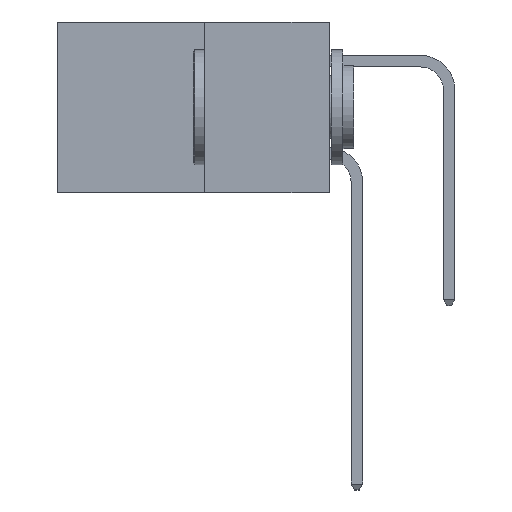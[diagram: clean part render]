
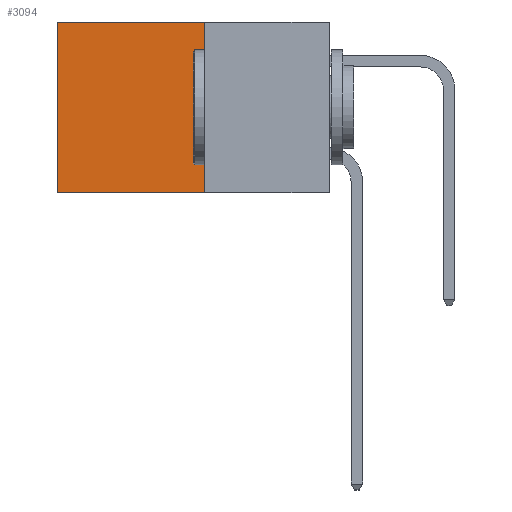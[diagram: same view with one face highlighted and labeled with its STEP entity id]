
A CAD part, left-side view. The second image highlights one B-rep face of the part: STEP entity #3094.
In plain terms, the highlighted planar face has unit normal (-1, 0, 0).
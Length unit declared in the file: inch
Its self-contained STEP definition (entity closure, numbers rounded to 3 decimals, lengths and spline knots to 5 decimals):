
#501 = DIRECTION ( 'NONE',  ( 0., 0., -1. ) ) ;
#2658 = ORIENTED_EDGE ( 'NONE', *, *, #6860, .T. ) ;
#2930 = VECTOR ( 'NONE', #501, 39.37008 ) ;
#3094 = ADVANCED_FACE ( 'NONE', ( #4518 ), #5995, .F. ) ;
#3196 = VERTEX_POINT ( 'NONE', #6927 ) ;
#3282 = LINE ( 'NONE', #6201, #2930 ) ;
#3519 = ORIENTED_EDGE ( 'NONE', *, *, #13353, .F. ) ;
#4063 = CARTESIAN_POINT ( 'NONE',  ( 0.277, 0.27, -0.37 ) ) ;
#4080 = CARTESIAN_POINT ( 'NONE',  ( 0.277, 0.27, 0. ) ) ;
#4437 = EDGE_LOOP ( 'NONE', ( #2658, #3519, #10215, #11850 ) ) ;
#4518 = FACE_OUTER_BOUND ( 'NONE', #4437, .T. ) ;
#4732 = DIRECTION ( 'NONE',  ( 0., 0., -1. ) ) ;
#4769 = DIRECTION ( 'NONE',  ( 1., 0., 0. ) ) ;
#4924 = LINE ( 'NONE', #4063, #14183 ) ;
#5316 = LINE ( 'NONE', #4080, #8425 ) ;
#5400 = VERTEX_POINT ( 'NONE', #12856 ) ;
#5650 = VECTOR ( 'NONE', #9365, 39.37008 ) ;
#5950 = CARTESIAN_POINT ( 'NONE',  ( 0.277, 0.27, -0.37 ) ) ;
#5995 = PLANE ( 'NONE',  #8934 ) ;
#6201 = CARTESIAN_POINT ( 'NONE',  ( 0.277, 0.59, -0.37 ) ) ;
#6860 = EDGE_CURVE ( 'NONE', #13932, #3196, #3282, .T. ) ;
#6927 = CARTESIAN_POINT ( 'NONE',  ( 0.277, 0.59, -0.37 ) ) ;
#8146 = CARTESIAN_POINT ( 'NONE',  ( 0.277, 0.59, 0. ) ) ;
#8181 = CARTESIAN_POINT ( 'NONE',  ( 0.277, 0.27, -0.37 ) ) ;
#8425 = VECTOR ( 'NONE', #13366, 39.37008 ) ;
#8934 = AXIS2_PLACEMENT_3D ( 'NONE', #5950, #4769, #4732 ) ;
#9365 = DIRECTION ( 'NONE',  ( 0., 0., -1. ) ) ;
#10215 = ORIENTED_EDGE ( 'NONE', *, *, #12403, .F. ) ;
#10831 = EDGE_CURVE ( 'NONE', #5400, #13932, #5316, .T. ) ;
#11850 = ORIENTED_EDGE ( 'NONE', *, *, #10831, .T. ) ;
#12181 = DIRECTION ( 'NONE',  ( 0., 1., 0. ) ) ;
#12227 = LINE ( 'NONE', #8181, #5650 ) ;
#12403 = EDGE_CURVE ( 'NONE', #5400, #12814, #12227, .T. ) ;
#12814 = VERTEX_POINT ( 'NONE', #14662 ) ;
#12856 = CARTESIAN_POINT ( 'NONE',  ( 0.277, 0.27, 0. ) ) ;
#13353 = EDGE_CURVE ( 'NONE', #12814, #3196, #4924, .T. ) ;
#13366 = DIRECTION ( 'NONE',  ( 0., 1., 0. ) ) ;
#13932 = VERTEX_POINT ( 'NONE', #8146 ) ;
#14183 = VECTOR ( 'NONE', #12181, 39.37008 ) ;
#14662 = CARTESIAN_POINT ( 'NONE',  ( 0.277, 0.27, -0.37 ) ) ;
